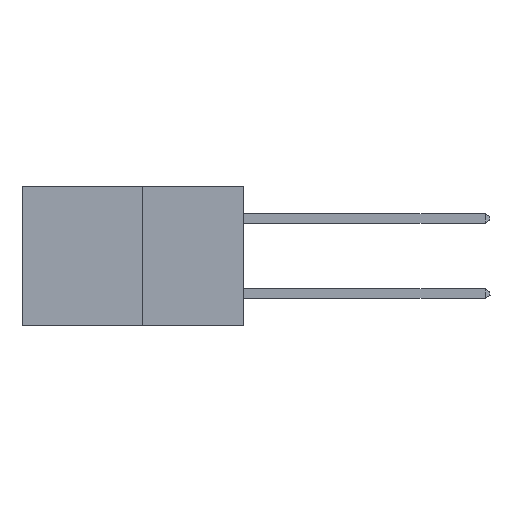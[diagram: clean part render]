
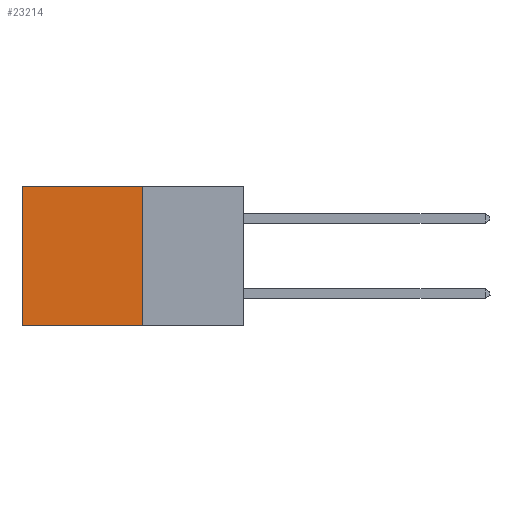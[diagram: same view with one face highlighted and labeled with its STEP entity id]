
A CAD part, left-side view. The second image highlights one B-rep face of the part: STEP entity #23214.
In plain terms, the highlighted planar face has unit normal (-1, 0, 0).
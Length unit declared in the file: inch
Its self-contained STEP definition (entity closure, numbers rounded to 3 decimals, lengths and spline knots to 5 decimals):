
#192 = LINE ( 'NONE', #11634, #15019 ) ;
#736 = LINE ( 'NONE', #20673, #10391 ) ;
#3663 = CARTESIAN_POINT ( 'NONE',  ( 0.277, 0.59, -0.37 ) ) ;
#4410 = PLANE ( 'NONE',  #14213 ) ;
#4764 = EDGE_CURVE ( 'NONE', #12963, #8882, #192, .T. ) ;
#5095 = VERTEX_POINT ( 'NONE', #3663 ) ;
#8293 = CARTESIAN_POINT ( 'NONE',  ( 0.277, 0.27, -0.37 ) ) ;
#8845 = CARTESIAN_POINT ( 'NONE',  ( 0.277, 0.27, 0. ) ) ;
#8882 = VERTEX_POINT ( 'NONE', #22261 ) ;
#8993 = LINE ( 'NONE', #8845, #9637 ) ;
#9637 = VECTOR ( 'NONE', #22353, 39.37008 ) ;
#10169 = ORIENTED_EDGE ( 'NONE', *, *, #17781, .T. ) ;
#10230 = DIRECTION ( 'NONE',  ( 0., 0., -1. ) ) ;
#10391 = VECTOR ( 'NONE', #11030, 39.37008 ) ;
#10985 = EDGE_CURVE ( 'NONE', #8882, #5095, #736, .T. ) ;
#11030 = DIRECTION ( 'NONE',  ( 0., 1., 0. ) ) ;
#11115 = DIRECTION ( 'NONE',  ( 0., 0., -1. ) ) ;
#11634 = CARTESIAN_POINT ( 'NONE',  ( 0.277, 0.27, -0.37 ) ) ;
#12963 = VERTEX_POINT ( 'NONE', #18901 ) ;
#14213 = AXIS2_PLACEMENT_3D ( 'NONE', #8293, #21826, #10230 ) ;
#14240 = EDGE_CURVE ( 'NONE', #12963, #17563, #8993, .T. ) ;
#14963 = LINE ( 'NONE', #21634, #24510 ) ;
#15019 = VECTOR ( 'NONE', #11115, 39.37008 ) ;
#15159 = CARTESIAN_POINT ( 'NONE',  ( 0.277, 0.59, 0. ) ) ;
#15301 = ORIENTED_EDGE ( 'NONE', *, *, #4764, .F. ) ;
#17563 = VERTEX_POINT ( 'NONE', #15159 ) ;
#17781 = EDGE_CURVE ( 'NONE', #17563, #5095, #14963, .T. ) ;
#18227 = EDGE_LOOP ( 'NONE', ( #10169, #19643, #15301, #18493 ) ) ;
#18493 = ORIENTED_EDGE ( 'NONE', *, *, #14240, .T. ) ;
#18901 = CARTESIAN_POINT ( 'NONE',  ( 0.277, 0.27, 0. ) ) ;
#19643 = ORIENTED_EDGE ( 'NONE', *, *, #10985, .F. ) ;
#20673 = CARTESIAN_POINT ( 'NONE',  ( 0.277, 0.27, -0.37 ) ) ;
#21634 = CARTESIAN_POINT ( 'NONE',  ( 0.277, 0.59, -0.37 ) ) ;
#21826 = DIRECTION ( 'NONE',  ( 1., 0., 0. ) ) ;
#22261 = CARTESIAN_POINT ( 'NONE',  ( 0.277, 0.27, -0.37 ) ) ;
#22353 = DIRECTION ( 'NONE',  ( 0., 1., 0. ) ) ;
#23059 = FACE_OUTER_BOUND ( 'NONE', #18227, .T. ) ;
#23214 = ADVANCED_FACE ( 'NONE', ( #23059 ), #4410, .F. ) ;
#23519 = DIRECTION ( 'NONE',  ( 0., 0., -1. ) ) ;
#24510 = VECTOR ( 'NONE', #23519, 39.37008 ) ;
